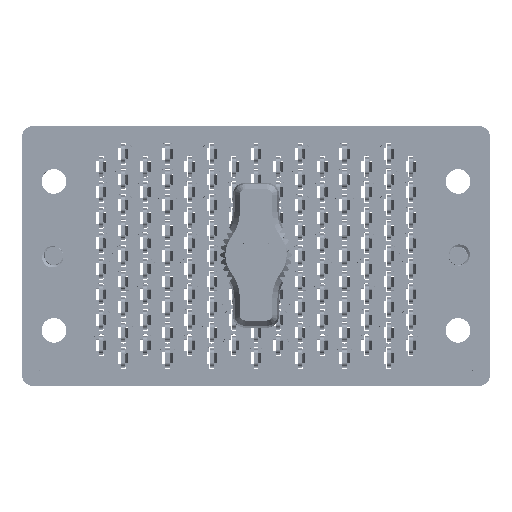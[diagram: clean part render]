
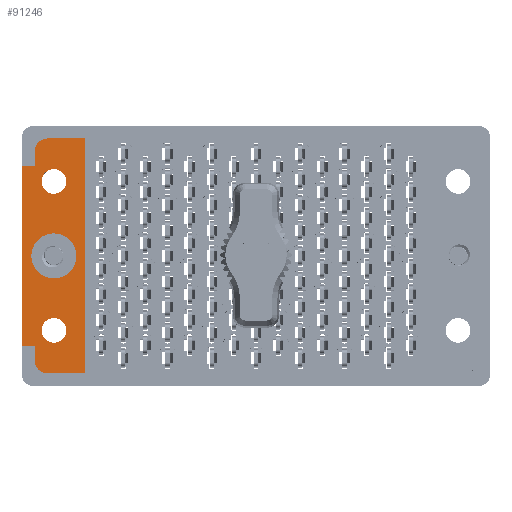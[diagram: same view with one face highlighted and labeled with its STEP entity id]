
A CAD part, top view. The second image highlights one B-rep face of the part: STEP entity #91246.
In plain terms, the highlighted planar face has unit normal (0, 0, 1).
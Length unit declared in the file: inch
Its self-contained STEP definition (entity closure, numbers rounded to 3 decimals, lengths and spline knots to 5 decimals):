
#564 = CARTESIAN_POINT ( 'NONE',  ( 0., -0.69, -0.117 ) ) ;
#1076 = CARTESIAN_POINT ( 'NONE',  ( -1.1875, 0., -0.117 ) ) ;
#1081 = LINE ( 'NONE', #101410, #65912 ) ;
#2419 = DIRECTION ( 'NONE',  ( 1., 0., 0. ) ) ;
#2889 = VERTEX_POINT ( 'NONE', #94523 ) ;
#3655 = CIRCLE ( 'NONE', #77234, 0.0725 ) ;
#5219 = DIRECTION ( 'NONE',  ( 1., 0., 0. ) ) ;
#6141 = CARTESIAN_POINT ( 'NONE',  ( -1.3, 0.5285, -0.117 ) ) ;
#6517 = AXIS2_PLACEMENT_3D ( 'NONE', #1076, #81945, #90811 ) ;
#7498 = VERTEX_POINT ( 'NONE', #115752 ) ;
#8817 = CIRCLE ( 'NONE', #50275, 0.0725 ) ;
#8995 = VERTEX_POINT ( 'NONE', #6141 ) ;
#9988 = ORIENTED_EDGE ( 'NONE', *, *, #51266, .F. ) ;
#10472 = ORIENTED_EDGE ( 'NONE', *, *, #69734, .T. ) ;
#12868 = CARTESIAN_POINT ( 'NONE',  ( 0., -0.5285, -0.117 ) ) ;
#13246 = CARTESIAN_POINT ( 'NONE',  ( -1.26, -0.4375, -0.117 ) ) ;
#14175 = VERTEX_POINT ( 'NONE', #69176 ) ;
#18012 = CARTESIAN_POINT ( 'NONE',  ( -1.1875, 0., -0.117 ) ) ;
#18266 = VERTEX_POINT ( 'NONE', #50447 ) ;
#18532 = AXIS2_PLACEMENT_3D ( 'NONE', #59245, #78691, #76395 ) ;
#20051 = LINE ( 'NONE', #564, #86270 ) ;
#20352 = CARTESIAN_POINT ( 'NONE',  ( -1.115, 0.4375, -0.117 ) ) ;
#20430 = DIRECTION ( 'NONE',  ( 0., 0., 1. ) ) ;
#20570 = VERTEX_POINT ( 'NONE', #102756 ) ;
#20669 = DIRECTION ( 'NONE',  ( 0., 0., 1. ) ) ;
#21455 = EDGE_LOOP ( 'NONE', ( #9988, #47200 ) ) ;
#21805 = DIRECTION ( 'NONE',  ( 1., 0., 0. ) ) ;
#22873 = AXIS2_PLACEMENT_3D ( 'NONE', #18012, #71147, #5219 ) ;
#23555 = CIRCLE ( 'NONE', #6517, 0.1325 ) ;
#24670 = CIRCLE ( 'NONE', #72019, 0.075 ) ;
#25613 = CARTESIAN_POINT ( 'NONE',  ( -1.005, 0.7625, -0.117 ) ) ;
#25887 = DIRECTION ( 'NONE',  ( 1., 0., 0. ) ) ;
#26223 = EDGE_CURVE ( 'NONE', #7498, #99337, #34336, .T. ) ;
#26797 = EDGE_CURVE ( 'NONE', #41237, #50125, #101364, .T. ) ;
#27507 = DIRECTION ( 'NONE',  ( 1., 0., 0. ) ) ;
#27529 = AXIS2_PLACEMENT_3D ( 'NONE', #46663, #20669, #21805 ) ;
#31752 = LINE ( 'NONE', #12868, #46843 ) ;
#31884 = CARTESIAN_POINT ( 'NONE',  ( -1.375, -0.5285, -0.117 ) ) ;
#33213 = DIRECTION ( 'NONE',  ( 0., 0., 1. ) ) ;
#34336 = LINE ( 'NONE', #70335, #46636 ) ;
#36379 = CARTESIAN_POINT ( 'NONE',  ( -1.225, -0.615, -0.117 ) ) ;
#37791 = PLANE ( 'NONE',  #27529 ) ;
#38765 = DIRECTION ( 'NONE',  ( 1., 0., 0. ) ) ;
#39452 = CIRCLE ( 'NONE', #109193, 0.0725 ) ;
#40197 = DIRECTION ( 'NONE',  ( 0., 0., 1. ) ) ;
#41237 = VERTEX_POINT ( 'NONE', #20352 ) ;
#41959 = EDGE_CURVE ( 'NONE', #65500, #98954, #51174, .T. ) ;
#44961 = ORIENTED_EDGE ( 'NONE', *, *, #113148, .F. ) ;
#46636 = VECTOR ( 'NONE', #106349, 39.37008 ) ;
#46663 = CARTESIAN_POINT ( 'NONE',  ( -1.375, -0.7625, -0.117 ) ) ;
#46767 = VECTOR ( 'NONE', #106919, 39.37008 ) ;
#46843 = VECTOR ( 'NONE', #110271, 39.37008 ) ;
#47200 = ORIENTED_EDGE ( 'NONE', *, *, #102544, .F. ) ;
#50125 = VERTEX_POINT ( 'NONE', #116356 ) ;
#50275 = AXIS2_PLACEMENT_3D ( 'NONE', #102926, #33213, #69227 ) ;
#50447 = CARTESIAN_POINT ( 'NONE',  ( -1.115, -0.4375, -0.117 ) ) ;
#50552 = AXIS2_PLACEMENT_3D ( 'NONE', #57317, #40197, #2419 ) ;
#51174 = CIRCLE ( 'NONE', #22873, 0.1325 ) ;
#51266 = EDGE_CURVE ( 'NONE', #76221, #18266, #8817, .T. ) ;
#54998 = CARTESIAN_POINT ( 'NONE',  ( -1.3, 0.615, -0.117 ) ) ;
#55465 = ORIENTED_EDGE ( 'NONE', *, *, #95258, .F. ) ;
#55947 = LINE ( 'NONE', #74243, #73483 ) ;
#56190 = EDGE_LOOP ( 'NONE', ( #44961, #65998 ) ) ;
#57317 = CARTESIAN_POINT ( 'NONE',  ( -1.1875, 0.4375, -0.117 ) ) ;
#58041 = EDGE_CURVE ( 'NONE', #50125, #41237, #3655, .T. ) ;
#59245 = CARTESIAN_POINT ( 'NONE',  ( -1.225, 0.615, -0.117 ) ) ;
#59711 = CARTESIAN_POINT ( 'NONE',  ( 0., 0.5285, -0.117 ) ) ;
#61626 = DIRECTION ( 'NONE',  ( 0., 1., 0. ) ) ;
#64269 = DIRECTION ( 'NONE',  ( 0., -1., 0. ) ) ;
#65500 = VERTEX_POINT ( 'NONE', #94828 ) ;
#65512 = FACE_BOUND ( 'NONE', #21455, .T. ) ;
#65631 = CIRCLE ( 'NONE', #18532, 0.075 ) ;
#65912 = VECTOR ( 'NONE', #64269, 39.37008 ) ;
#65998 = ORIENTED_EDGE ( 'NONE', *, *, #41959, .F. ) ;
#66487 = VERTEX_POINT ( 'NONE', #75089 ) ;
#66531 = DIRECTION ( 'NONE',  ( 0., -1., 0. ) ) ;
#69176 = CARTESIAN_POINT ( 'NONE',  ( -1.3, -0.5285, -0.117 ) ) ;
#69227 = DIRECTION ( 'NONE',  ( 1., 0., 0. ) ) ;
#69734 = EDGE_CURVE ( 'NONE', #99337, #108720, #65631, .T. ) ;
#70324 = LINE ( 'NONE', #59711, #46767 ) ;
#70335 = CARTESIAN_POINT ( 'NONE',  ( 0., 0.69, -0.117 ) ) ;
#70613 = CARTESIAN_POINT ( 'NONE',  ( -1.375, 0.7625, -0.117 ) ) ;
#71147 = DIRECTION ( 'NONE',  ( 0., 0., 1. ) ) ;
#71837 = VERTEX_POINT ( 'NONE', #101541 ) ;
#72019 = AXIS2_PLACEMENT_3D ( 'NONE', #36379, #20430, #27507 ) ;
#72321 = EDGE_CURVE ( 'NONE', #108720, #8995, #1081, .T. ) ;
#73483 = VECTOR ( 'NONE', #66531, 39.37008 ) ;
#73597 = CARTESIAN_POINT ( 'NONE',  ( -1.1875, -0.4375, -0.117 ) ) ;
#74243 = CARTESIAN_POINT ( 'NONE',  ( -1.3, 0., -0.117 ) ) ;
#74590 = EDGE_CURVE ( 'NONE', #14175, #20570, #55947, .T. ) ;
#75089 = CARTESIAN_POINT ( 'NONE',  ( -1.005, -0.69, -0.117 ) ) ;
#75622 = VERTEX_POINT ( 'NONE', #31884 ) ;
#75828 = EDGE_LOOP ( 'NONE', ( #99550, #92391 ) ) ;
#76221 = VERTEX_POINT ( 'NONE', #13246 ) ;
#76395 = DIRECTION ( 'NONE',  ( 1., 0., 0. ) ) ;
#76662 = ORIENTED_EDGE ( 'NONE', *, *, #26223, .T. ) ;
#77234 = AXIS2_PLACEMENT_3D ( 'NONE', #115588, #106750, #25887 ) ;
#78276 = EDGE_CURVE ( 'NONE', #71837, #75622, #107214, .T. ) ;
#78691 = DIRECTION ( 'NONE',  ( 0., 0., 1. ) ) ;
#78814 = EDGE_LOOP ( 'NONE', ( #76662, #10472, #86576, #84564, #89123, #55465, #95377, #116712, #101211, #85352 ) ) ;
#81945 = DIRECTION ( 'NONE',  ( 0., 0., 1. ) ) ;
#82605 = DIRECTION ( 'NONE',  ( -1., 0., 0. ) ) ;
#83608 = DIRECTION ( 'NONE',  ( 0., 0., 1. ) ) ;
#84564 = ORIENTED_EDGE ( 'NONE', *, *, #94627, .T. ) ;
#84713 = EDGE_CURVE ( 'NONE', #20570, #2889, #24670, .T. ) ;
#85352 = ORIENTED_EDGE ( 'NONE', *, *, #94212, .T. ) ;
#86270 = VECTOR ( 'NONE', #82605, 39.37008 ) ;
#86576 = ORIENTED_EDGE ( 'NONE', *, *, #72321, .T. ) ;
#88076 = VECTOR ( 'NONE', #61626, 39.37008 ) ;
#88903 = DIRECTION ( 'NONE',  ( 0., -1., 0. ) ) ;
#89123 = ORIENTED_EDGE ( 'NONE', *, *, #78276, .T. ) ;
#90811 = DIRECTION ( 'NONE',  ( 1., 0., 0. ) ) ;
#91246 = ADVANCED_FACE ( 'NONE', ( #102080, #65512, #91498, #110933 ), #37791, .T. ) ;
#91498 = FACE_BOUND ( 'NONE', #56190, .T. ) ;
#92391 = ORIENTED_EDGE ( 'NONE', *, *, #26797, .F. ) ;
#92625 = CARTESIAN_POINT ( 'NONE',  ( -1.225, 0.69, -0.117 ) ) ;
#94212 = EDGE_CURVE ( 'NONE', #66487, #7498, #106484, .T. ) ;
#94523 = CARTESIAN_POINT ( 'NONE',  ( -1.225, -0.69, -0.117 ) ) ;
#94627 = EDGE_CURVE ( 'NONE', #8995, #71837, #70324, .T. ) ;
#94828 = CARTESIAN_POINT ( 'NONE',  ( -1.32, 0., -0.117 ) ) ;
#95258 = EDGE_CURVE ( 'NONE', #14175, #75622, #31752, .T. ) ;
#95377 = ORIENTED_EDGE ( 'NONE', *, *, #74590, .T. ) ;
#98954 = VERTEX_POINT ( 'NONE', #110459 ) ;
#99337 = VERTEX_POINT ( 'NONE', #92625 ) ;
#99360 = EDGE_CURVE ( 'NONE', #66487, #2889, #20051, .T. ) ;
#99550 = ORIENTED_EDGE ( 'NONE', *, *, #58041, .F. ) ;
#101211 = ORIENTED_EDGE ( 'NONE', *, *, #99360, .F. ) ;
#101364 = CIRCLE ( 'NONE', #50552, 0.0725 ) ;
#101410 = CARTESIAN_POINT ( 'NONE',  ( -1.3, 0., -0.117 ) ) ;
#101541 = CARTESIAN_POINT ( 'NONE',  ( -1.375, 0.5285, -0.117 ) ) ;
#102080 = FACE_BOUND ( 'NONE', #75828, .T. ) ;
#102544 = EDGE_CURVE ( 'NONE', #18266, #76221, #39452, .T. ) ;
#102756 = CARTESIAN_POINT ( 'NONE',  ( -1.3, -0.615, -0.117 ) ) ;
#102926 = CARTESIAN_POINT ( 'NONE',  ( -1.1875, -0.4375, -0.117 ) ) ;
#106349 = DIRECTION ( 'NONE',  ( -1., 0., 0. ) ) ;
#106484 = LINE ( 'NONE', #25613, #88076 ) ;
#106750 = DIRECTION ( 'NONE',  ( 0., 0., 1. ) ) ;
#106919 = DIRECTION ( 'NONE',  ( -1., 0., 0. ) ) ;
#107214 = LINE ( 'NONE', #70613, #113639 ) ;
#108720 = VERTEX_POINT ( 'NONE', #54998 ) ;
#109193 = AXIS2_PLACEMENT_3D ( 'NONE', #73597, #83608, #38765 ) ;
#110271 = DIRECTION ( 'NONE',  ( -1., 0., 0. ) ) ;
#110459 = CARTESIAN_POINT ( 'NONE',  ( -1.055, 0., -0.117 ) ) ;
#110933 = FACE_OUTER_BOUND ( 'NONE', #78814, .T. ) ;
#113148 = EDGE_CURVE ( 'NONE', #98954, #65500, #23555, .T. ) ;
#113639 = VECTOR ( 'NONE', #88903, 39.37008 ) ;
#115588 = CARTESIAN_POINT ( 'NONE',  ( -1.1875, 0.4375, -0.117 ) ) ;
#115752 = CARTESIAN_POINT ( 'NONE',  ( -1.005, 0.69, -0.117 ) ) ;
#116356 = CARTESIAN_POINT ( 'NONE',  ( -1.26, 0.4375, -0.117 ) ) ;
#116712 = ORIENTED_EDGE ( 'NONE', *, *, #84713, .T. ) ;
